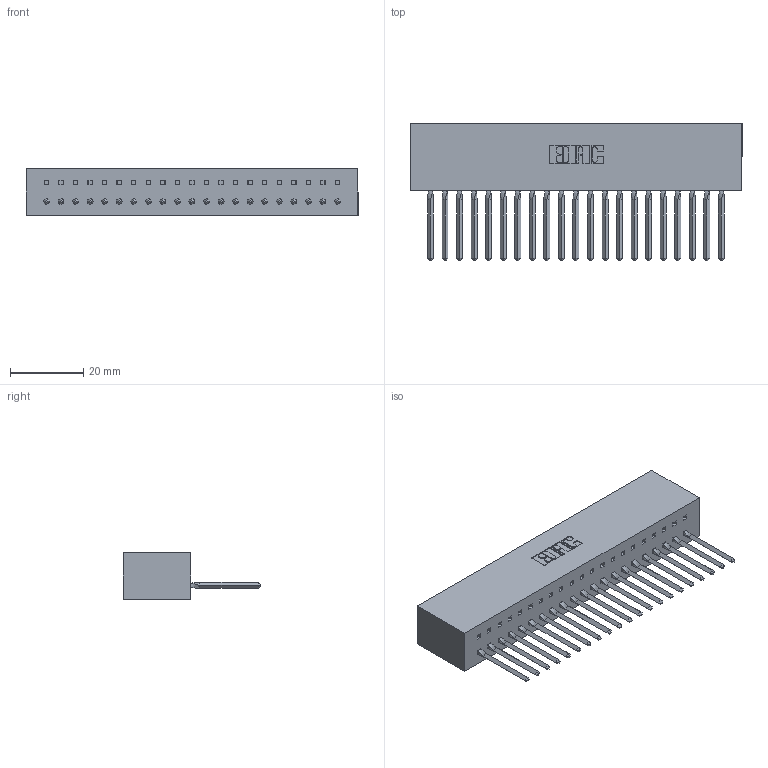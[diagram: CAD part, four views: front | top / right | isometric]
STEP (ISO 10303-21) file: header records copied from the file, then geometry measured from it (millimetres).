
FILE_DESCRIPTION (( 'STEP AP203' ), '1' );
FILE_NAME ('317-021-541-601.STEP', '2020-02-27T17:02:13', ( '' ), ( '' ), 'SwSTEP 2.0', 'SolidWorks 2016', '' );
FILE_SCHEMA (( 'CONFIG_CONTROL_DESIGN' ));
Length unit declared in the file: inch
Products named in the file (3): 317-021-541-601; 317-290-002_541; 317 Part_Lugless
Assembly tree (22 placements, depth 2):
  317-021-541-601
    317 Part_Lugless
    317-290-002_541  x21
Bounding box: 90.42 x 37.34 x 12.7 mm (x, y, z)
Volume: 15723.8 mm3; surface area: 21712.4 mm2
Topology: 22 solids, 22 shells, 3282 faces, 9353 edges, 6080 vertices
Faces by surface type: plane 2654, cylinder 544, bspline 84
Entity records: 33752 total; most frequent: CARTESIAN_POINT 6632, ORIENTED_EDGE 5906, DIRECTION 4827, EDGE_CURVE 2953, LINE 2597, VECTOR 2597, VERTEX_POINT 1960, AXIS2_PLACEMENT_3D 1115
